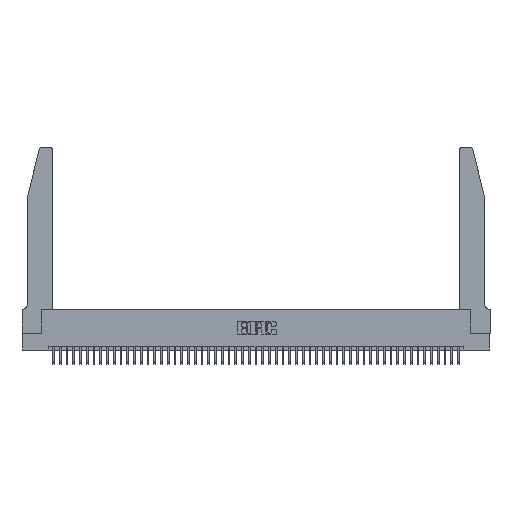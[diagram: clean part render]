
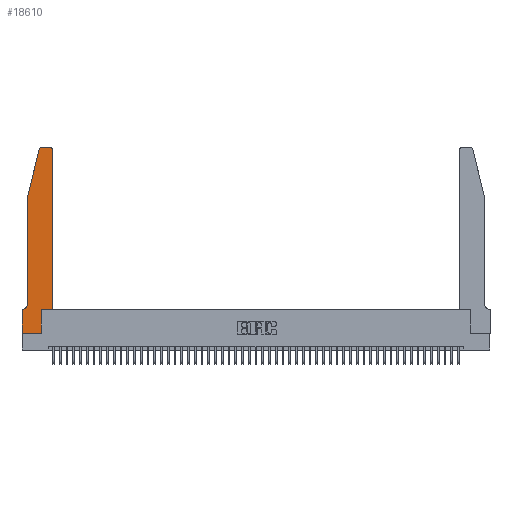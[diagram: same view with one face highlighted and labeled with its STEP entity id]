
A CAD part, top view. The second image highlights one B-rep face of the part: STEP entity #18610.
In plain terms, the highlighted planar face has unit normal (0, 0, 1).
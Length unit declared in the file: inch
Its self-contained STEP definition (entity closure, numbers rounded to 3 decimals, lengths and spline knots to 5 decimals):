
#194 = ORIENTED_EDGE ( 'NONE', *, *, #30722, .T. ) ;
#744 = CARTESIAN_POINT ( 'NONE',  ( 0.0755, 2., 0.37 ) ) ;
#975 = CARTESIAN_POINT ( 'NONE',  ( 0.2865, 0.35, 0.37 ) ) ;
#1432 = EDGE_CURVE ( 'NONE', #26130, #20535, #46337, .T. ) ;
#4120 = VECTOR ( 'NONE', #50934, 39.37008 ) ;
#4722 = CARTESIAN_POINT ( 'NONE',  ( 0.0755, 2., 0.37 ) ) ;
#5239 = DIRECTION ( 'NONE',  ( -1., 0., 0. ) ) ;
#5528 = AXIS2_PLACEMENT_3D ( 'NONE', #6667, #50692, #7173 ) ;
#5798 = CARTESIAN_POINT ( 'NONE',  ( 0.4205, 2.75, 0.37 ) ) ;
#5908 = CARTESIAN_POINT ( 'NONE',  ( 0.4205, 2.72, 0.37 ) ) ;
#6157 = VERTEX_POINT ( 'NONE', #50479 ) ;
#6667 = CARTESIAN_POINT ( 'NONE',  ( 0.284, 2.72, 0.37 ) ) ;
#7173 = DIRECTION ( 'NONE',  ( 1., 0., 0. ) ) ;
#7320 = CARTESIAN_POINT ( 'NONE',  ( 0.4505, 0.35, 0.37 ) ) ;
#7471 = CARTESIAN_POINT ( 'NONE',  ( 0., 0., 0.37 ) ) ;
#7701 = CARTESIAN_POINT ( 'NONE',  ( 0.0755, 2., 0.37 ) ) ;
#8646 = ORIENTED_EDGE ( 'NONE', *, *, #44286, .T. ) ;
#10627 = CARTESIAN_POINT ( 'NONE',  ( 0.0755, 0.35, 0.37 ) ) ;
#10681 = CARTESIAN_POINT ( 'NONE',  ( 0.0755, 0.42, 0.37 ) ) ;
#11191 = CIRCLE ( 'NONE', #5528, 0.03 ) ;
#12266 = DIRECTION ( 'NONE',  ( 0., -1., 0. ) ) ;
#12779 = LINE ( 'NONE', #7701, #49021 ) ;
#12941 = DIRECTION ( 'NONE',  ( 0., 0., 1. ) ) ;
#13288 = PLANE ( 'NONE',  #22640 ) ;
#13657 = VECTOR ( 'NONE', #5239, 39.37008 ) ;
#14199 = AXIS2_PLACEMENT_3D ( 'NONE', #5908, #30220, #33694 ) ;
#14956 = EDGE_CURVE ( 'NONE', #20535, #51029, #25911, .T. ) ;
#15273 = VECTOR ( 'NONE', #44075, 39.37008 ) ;
#15384 = DIRECTION ( 'NONE',  ( 1., 0., 0. ) ) ;
#16374 = ORIENTED_EDGE ( 'NONE', *, *, #1432, .T. ) ;
#16990 = VERTEX_POINT ( 'NONE', #39461 ) ;
#17288 = LINE ( 'NONE', #10627, #4120 ) ;
#17561 = LINE ( 'NONE', #7320, #19473 ) ;
#17863 = CARTESIAN_POINT ( 'NONE',  ( 0.0055, 0.42, 0.37 ) ) ;
#18136 = ORIENTED_EDGE ( 'NONE', *, *, #24988, .T. ) ;
#18545 = EDGE_CURVE ( 'NONE', #36665, #33397, #22432, .T. ) ;
#18610 = ADVANCED_FACE ( 'NONE', ( #31788 ), #13288, .T. ) ;
#19284 = CARTESIAN_POINT ( 'NONE',  ( 0., 0., 0.37 ) ) ;
#19473 = VECTOR ( 'NONE', #15384, 39.37008 ) ;
#20117 = EDGE_LOOP ( 'NONE', ( #24146, #27066, #8646, #24507, #45350, #18136, #34556, #16374, #26522, #43489, #194, #50456 ) ) ;
#20535 = VERTEX_POINT ( 'NONE', #30228 ) ;
#21502 = CARTESIAN_POINT ( 'NONE',  ( 0.4505, 0.35, 0.37 ) ) ;
#21884 = DIRECTION ( 'NONE',  ( -1., 0., 0. ) ) ;
#22086 = CARTESIAN_POINT ( 'NONE',  ( 0.25487, 2.72718, 0.37 ) ) ;
#22432 = LINE ( 'NONE', #48571, #13657 ) ;
#22440 = DIRECTION ( 'NONE',  ( 0., -1., 0. ) ) ;
#22492 = LINE ( 'NONE', #50030, #37466 ) ;
#22640 = AXIS2_PLACEMENT_3D ( 'NONE', #44710, #12941, #24826 ) ;
#23573 = EDGE_CURVE ( 'NONE', #16990, #26130, #22492, .T. ) ;
#24146 = ORIENTED_EDGE ( 'NONE', *, *, #18545, .T. ) ;
#24507 = ORIENTED_EDGE ( 'NONE', *, *, #26246, .T. ) ;
#24826 = DIRECTION ( 'NONE',  ( 1., 0., 0. ) ) ;
#24988 = EDGE_CURVE ( 'NONE', #36139, #16990, #17288, .T. ) ;
#25911 = LINE ( 'NONE', #975, #15273 ) ;
#26130 = VERTEX_POINT ( 'NONE', #19284 ) ;
#26141 = VECTOR ( 'NONE', #27737, 39.37008 ) ;
#26246 = EDGE_CURVE ( 'NONE', #41193, #35006, #12779, .T. ) ;
#26522 = ORIENTED_EDGE ( 'NONE', *, *, #14956, .T. ) ;
#27066 = ORIENTED_EDGE ( 'NONE', *, *, #42755, .T. ) ;
#27269 = VECTOR ( 'NONE', #33041, 39.37008 ) ;
#27737 = DIRECTION ( 'NONE',  ( 0., 1., 0. ) ) ;
#30220 = DIRECTION ( 'NONE',  ( 0., 0., 1. ) ) ;
#30228 = CARTESIAN_POINT ( 'NONE',  ( 0.2865, 0., 0.37 ) ) ;
#30722 = EDGE_CURVE ( 'NONE', #44374, #6157, #47380, .T. ) ;
#30768 = CARTESIAN_POINT ( 'NONE',  ( 0.284, 2.75, 0.37 ) ) ;
#31498 = CIRCLE ( 'NONE', #33159, 0.07 ) ;
#31663 = VERTEX_POINT ( 'NONE', #22086 ) ;
#31788 = FACE_OUTER_BOUND ( 'NONE', #20117, .T. ) ;
#33041 = DIRECTION ( 'NONE',  ( -0.239, -0.971, 0. ) ) ;
#33159 = AXIS2_PLACEMENT_3D ( 'NONE', #17863, #45802, #21884 ) ;
#33278 = CIRCLE ( 'NONE', #14199, 0.03 ) ;
#33397 = VERTEX_POINT ( 'NONE', #30768 ) ;
#33694 = DIRECTION ( 'NONE',  ( 1., 0., 0. ) ) ;
#34216 = CARTESIAN_POINT ( 'NONE',  ( 0.2865, 0.35, 0.37 ) ) ;
#34556 = ORIENTED_EDGE ( 'NONE', *, *, #23573, .T. ) ;
#35006 = VERTEX_POINT ( 'NONE', #10681 ) ;
#35594 = DIRECTION ( 'NONE',  ( 1., 0., 0. ) ) ;
#36139 = VERTEX_POINT ( 'NONE', #37289 ) ;
#36665 = VERTEX_POINT ( 'NONE', #5798 ) ;
#36969 = EDGE_CURVE ( 'NONE', #51029, #44374, #17561, .T. ) ;
#37289 = CARTESIAN_POINT ( 'NONE',  ( 0.0055, 0.35, 0.37 ) ) ;
#37466 = VECTOR ( 'NONE', #22440, 39.37008 ) ;
#39461 = CARTESIAN_POINT ( 'NONE',  ( 0., 0.35, 0.37 ) ) ;
#40175 = EDGE_CURVE ( 'NONE', #6157, #36665, #33278, .T. ) ;
#41193 = VERTEX_POINT ( 'NONE', #744 ) ;
#42244 = LINE ( 'NONE', #4722, #27269 ) ;
#42755 = EDGE_CURVE ( 'NONE', #33397, #31663, #11191, .T. ) ;
#43489 = ORIENTED_EDGE ( 'NONE', *, *, #36969, .T. ) ;
#44075 = DIRECTION ( 'NONE',  ( 0., 1., 0. ) ) ;
#44286 = EDGE_CURVE ( 'NONE', #31663, #41193, #42244, .T. ) ;
#44374 = VERTEX_POINT ( 'NONE', #21502 ) ;
#44710 = CARTESIAN_POINT ( 'NONE',  ( 0., 0.35, 0.37 ) ) ;
#45053 = VECTOR ( 'NONE', #35594, 39.37008 ) ;
#45350 = ORIENTED_EDGE ( 'NONE', *, *, #50307, .T. ) ;
#45802 = DIRECTION ( 'NONE',  ( 0., 0., -1. ) ) ;
#46337 = LINE ( 'NONE', #7471, #45053 ) ;
#47325 = CARTESIAN_POINT ( 'NONE',  ( 0.4505, 0.35, 0.37 ) ) ;
#47380 = LINE ( 'NONE', #47325, #26141 ) ;
#48571 = CARTESIAN_POINT ( 'NONE',  ( 0.2605, 2.75, 0.37 ) ) ;
#49021 = VECTOR ( 'NONE', #12266, 39.37008 ) ;
#50030 = CARTESIAN_POINT ( 'NONE',  ( 0., 0., 0.37 ) ) ;
#50307 = EDGE_CURVE ( 'NONE', #35006, #36139, #31498, .T. ) ;
#50456 = ORIENTED_EDGE ( 'NONE', *, *, #40175, .T. ) ;
#50479 = CARTESIAN_POINT ( 'NONE',  ( 0.4505, 2.72, 0.37 ) ) ;
#50692 = DIRECTION ( 'NONE',  ( 0., 0., 1. ) ) ;
#50934 = DIRECTION ( 'NONE',  ( -1., 0., 0. ) ) ;
#51029 = VERTEX_POINT ( 'NONE', #34216 ) ;
